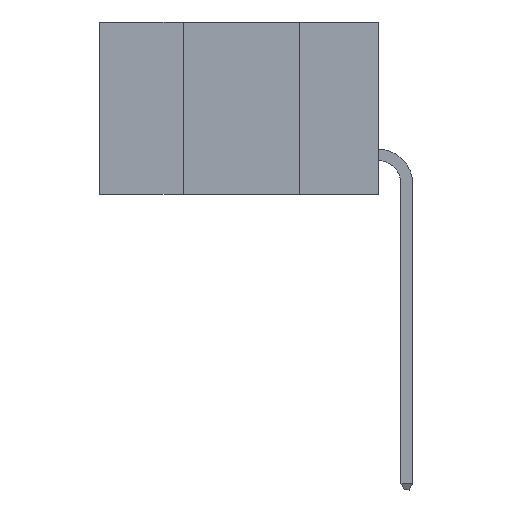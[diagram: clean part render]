
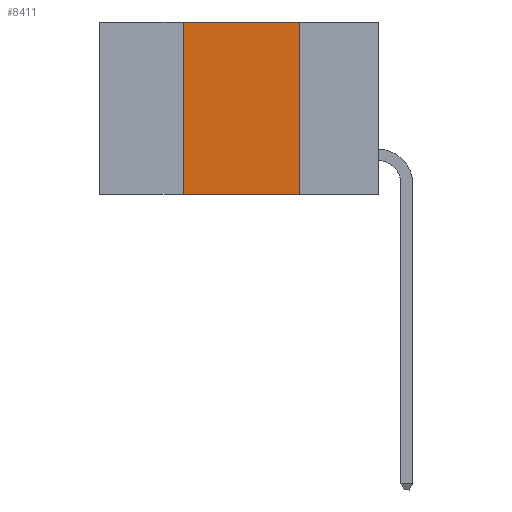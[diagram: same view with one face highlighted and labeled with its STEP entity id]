
A CAD part, left-side view. The second image highlights one B-rep face of the part: STEP entity #8411.
In plain terms, the highlighted planar face has unit normal (-1, 0, 0).
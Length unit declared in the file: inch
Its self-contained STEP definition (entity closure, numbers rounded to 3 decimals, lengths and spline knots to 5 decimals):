
#41 = LINE ( 'NONE', #6540, #6079 ) ;
#77 = VECTOR ( 'NONE', #6013, 39.37008 ) ;
#345 = LINE ( 'NONE', #9510, #77 ) ;
#467 = LINE ( 'NONE', #8591, #7218 ) ;
#795 = CARTESIAN_POINT ( 'NONE',  ( 0., 0.6, 0. ) ) ;
#843 = DIRECTION ( 'NONE',  ( 0., 0., 1. ) ) ;
#1351 = DIRECTION ( 'NONE',  ( 0., -1., 0. ) ) ;
#1724 = CARTESIAN_POINT ( 'NONE',  ( 0., 0.42, 0. ) ) ;
#2016 = CARTESIAN_POINT ( 'NONE',  ( 0., 0.17, 0. ) ) ;
#2203 = EDGE_CURVE ( 'NONE', #10118, #10854, #10074, .T. ) ;
#2372 = EDGE_CURVE ( 'NONE', #10757, #10854, #345, .T. ) ;
#2589 = ORIENTED_EDGE ( 'NONE', *, *, #2203, .F. ) ;
#3177 = VECTOR ( 'NONE', #8303, 39.37008 ) ;
#3314 = DIRECTION ( 'NONE',  ( 0., 0., -1. ) ) ;
#3715 = ORIENTED_EDGE ( 'NONE', *, *, #7789, .F. ) ;
#3758 = AXIS2_PLACEMENT_3D ( 'NONE', #795, #6928, #3314 ) ;
#3850 = CARTESIAN_POINT ( 'NONE',  ( 0., 0.17, -0.37 ) ) ;
#4826 = CARTESIAN_POINT ( 'NONE',  ( 0., 0.17, 0. ) ) ;
#4916 = ORIENTED_EDGE ( 'NONE', *, *, #2372, .T. ) ;
#6013 = DIRECTION ( 'NONE',  ( 0., -1., 0. ) ) ;
#6079 = VECTOR ( 'NONE', #1351, 39.37008 ) ;
#6540 = CARTESIAN_POINT ( 'NONE',  ( 0., 0.6, 0. ) ) ;
#6928 = DIRECTION ( 'NONE',  ( 1., 0., 0. ) ) ;
#7204 = FACE_OUTER_BOUND ( 'NONE', #7771, .T. ) ;
#7218 = VECTOR ( 'NONE', #843, 39.37008 ) ;
#7771 = EDGE_LOOP ( 'NONE', ( #2589, #11156, #3715, #4916 ) ) ;
#7789 = EDGE_CURVE ( 'NONE', #10757, #8963, #467, .T. ) ;
#8303 = DIRECTION ( 'NONE',  ( 0., 0., -1. ) ) ;
#8411 = ADVANCED_FACE ( 'NONE', ( #7204 ), #10272, .F. ) ;
#8591 = CARTESIAN_POINT ( 'NONE',  ( 0., 0.42, 0. ) ) ;
#8844 = EDGE_CURVE ( 'NONE', #8963, #10118, #41, .T. ) ;
#8963 = VERTEX_POINT ( 'NONE', #1724 ) ;
#9510 = CARTESIAN_POINT ( 'NONE',  ( 0., 0.6, -0.37 ) ) ;
#9796 = CARTESIAN_POINT ( 'NONE',  ( 0., 0.42, -0.37 ) ) ;
#10074 = LINE ( 'NONE', #4826, #3177 ) ;
#10118 = VERTEX_POINT ( 'NONE', #2016 ) ;
#10272 = PLANE ( 'NONE',  #3758 ) ;
#10757 = VERTEX_POINT ( 'NONE', #9796 ) ;
#10854 = VERTEX_POINT ( 'NONE', #3850 ) ;
#11156 = ORIENTED_EDGE ( 'NONE', *, *, #8844, .F. ) ;
